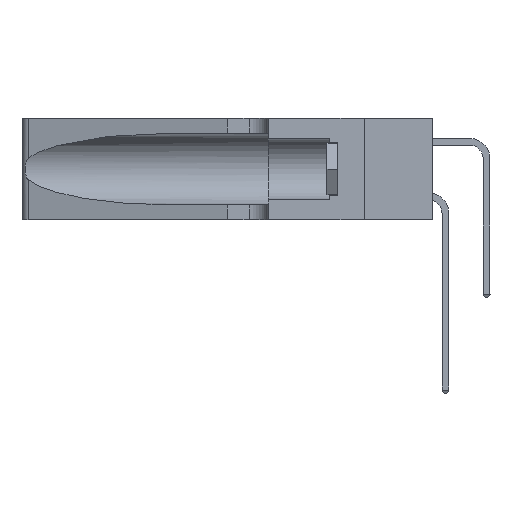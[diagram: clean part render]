
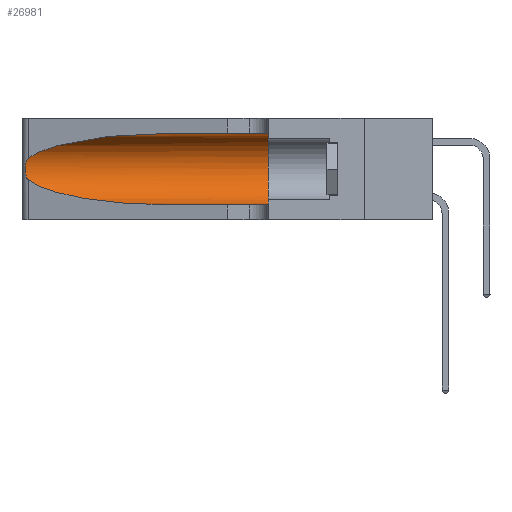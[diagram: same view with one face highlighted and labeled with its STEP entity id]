
A CAD part, left-side view. The second image highlights one B-rep face of the part: STEP entity #26981.
In plain terms, the highlighted cylindrical face has radius 3.308 mm (diameter 6.617 mm), a partial arc.
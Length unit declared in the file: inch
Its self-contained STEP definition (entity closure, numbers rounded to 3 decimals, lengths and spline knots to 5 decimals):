
#439 = CARTESIAN_POINT ( 'NONE',  ( 0.1305, 0.35, 0.185 ) ) ;
#847 = CARTESIAN_POINT ( 'NONE',  ( 0.25555, 1.22994, 0.2215 ) ) ;
#937 = CARTESIAN_POINT ( 'NONE',  ( 0.26017, 1.23833, 0.17102 ) ) ;
#1158 = CIRCLE ( 'NONE', #15803, 0.13025 ) ;
#1574 = CARTESIAN_POINT ( 'NONE',  ( 0.1305, 1.61858, 0.31525 ) ) ;
#1916 = CARTESIAN_POINT ( 'NONE',  ( 0.2373, 1.15595, 0.08982 ) ) ;
#1988 = ORIENTED_EDGE ( 'NONE', *, *, #2039, .T. ) ;
#2039 = EDGE_CURVE ( 'NONE', #26593, #8011, #4133, .T. ) ;
#2367 = ORIENTED_EDGE ( 'NONE', *, *, #3461, .T. ) ;
#2606 = EDGE_CURVE ( 'NONE', #6493, #22033, #1158, .T. ) ;
#2613 = DIRECTION ( 'NONE',  ( 0., 0., 1. ) ) ;
#2616 = CARTESIAN_POINT ( 'NONE',  ( 0.1305, 0.72297, 0.31525 ) ) ;
#3126 = CARTESIAN_POINT ( 'NONE',  ( 0.25789, 1.23486, 0.15765 ) ) ;
#3461 = EDGE_CURVE ( 'NONE', #25106, #22033, #8865, .T. ) ;
#4133 = B_SPLINE_CURVE_WITH_KNOTS ( 'NONE', 3,
 ( #22318, #847, #7370, #9510, #24423, #11702, #26543, #13853, #937, #15999, #3126, #18124, #5297, #20237 ),
 .UNSPECIFIED., .F., .F.,
 ( 4, 2, 2, 2, 2, 2, 4 ),
 ( 0., 0.00027, 0.00053, 0.00107, 0.0016, 0.00187, 0.00214 ),
 .UNSPECIFIED. ) ;
#4388 = ORIENTED_EDGE ( 'NONE', *, *, #7246, .T. ) ;
#4979 =( BOUNDED_CURVE ( )  B_SPLINE_CURVE ( 3, ( #8338, #1916, #19069, #6282 ),
 .UNSPECIFIED., .F., .F. ) 
 B_SPLINE_CURVE_WITH_KNOTS ( ( 4, 4 ),
 ( 3.44316, 4.71239 ),
 .UNSPECIFIED. ) 
 CURVE ( )  GEOMETRIC_REPRESENTATION_ITEM ( )  RATIONAL_B_SPLINE_CURVE ( ( 1., 0.87, 0.87, 1. ) ) 
 REPRESENTATION_ITEM ( '' )  );
#5297 = CARTESIAN_POINT ( 'NONE',  ( 0.25555, 1.22993, 0.14849 ) ) ;
#5604 = VECTOR ( 'NONE', #16625, 39.37008 ) ;
#5694 = CARTESIAN_POINT ( 'NONE',  ( 0.1305, 0.35, 0.05475 ) ) ;
#6282 = CARTESIAN_POINT ( 'NONE',  ( 0.1305, 0.72297, 0.05475 ) ) ;
#6493 = VERTEX_POINT ( 'NONE', #25666 ) ;
#6662 = AXIS2_PLACEMENT_3D ( 'NONE', #27594, #27686, #14990 ) ;
#7246 = EDGE_CURVE ( 'NONE', #23212, #26593, #12064, .T. ) ;
#7370 = CARTESIAN_POINT ( 'NONE',  ( 0.25639, 1.23184, 0.21858 ) ) ;
#8011 = VERTEX_POINT ( 'NONE', #9977 ) ;
#8197 = VECTOR ( 'NONE', #12387, 39.37008 ) ;
#8338 = CARTESIAN_POINT ( 'NONE',  ( 0.25487, 1.22718, 0.14631 ) ) ;
#8865 = LINE ( 'NONE', #10211, #8197 ) ;
#9374 = CARTESIAN_POINT ( 'NONE',  ( 0.25487, 1.22718, 0.22369 ) ) ;
#9510 = CARTESIAN_POINT ( 'NONE',  ( 0.25787, 1.23484, 0.2124 ) ) ;
#9977 = CARTESIAN_POINT ( 'NONE',  ( 0.25487, 1.22718, 0.14631 ) ) ;
#10211 = CARTESIAN_POINT ( 'NONE',  ( 0.1305, 1.61858, 0.05475 ) ) ;
#11135 = CARTESIAN_POINT ( 'NONE',  ( 0.2373, 1.15595, 0.28018 ) ) ;
#11506 = ORIENTED_EDGE ( 'NONE', *, *, #26190, .F. ) ;
#11702 = CARTESIAN_POINT ( 'NONE',  ( 0.26018, 1.23835, 0.19895 ) ) ;
#11724 = EDGE_CURVE ( 'NONE', #8011, #25106, #4979, .T. ) ;
#11952 = CYLINDRICAL_SURFACE ( 'NONE', #6662, 0.13025 ) ;
#12064 =( BOUNDED_CURVE ( )  B_SPLINE_CURVE ( 3, ( #21747, #23882, #11135, #25993 ),
 .UNSPECIFIED., .F., .F. ) 
 B_SPLINE_CURVE_WITH_KNOTS ( ( 4, 4 ),
 ( 1.5708, 2.84003 ),
 .UNSPECIFIED. ) 
 CURVE ( )  GEOMETRIC_REPRESENTATION_ITEM ( )  RATIONAL_B_SPLINE_CURVE ( ( 1., 0.87, 0.87, 1. ) ) 
 REPRESENTATION_ITEM ( '' )  );
#12387 = DIRECTION ( 'NONE',  ( 0., -1., 0. ) ) ;
#12666 = ORIENTED_EDGE ( 'NONE', *, *, #2606, .F. ) ;
#13853 = CARTESIAN_POINT ( 'NONE',  ( 0.26075, 1.23896, 0.178 ) ) ;
#14990 = DIRECTION ( 'NONE',  ( 0., 0., -1. ) ) ;
#15486 = DIRECTION ( 'NONE',  ( 0., 1., 0. ) ) ;
#15803 = AXIS2_PLACEMENT_3D ( 'NONE', #439, #15486, #2613 ) ;
#15999 = CARTESIAN_POINT ( 'NONE',  ( 0.25856, 1.23593, 0.16098 ) ) ;
#16625 = DIRECTION ( 'NONE',  ( 0., -1., 0. ) ) ;
#16942 = EDGE_LOOP ( 'NONE', ( #4388, #1988, #22375, #2367, #12666, #11506 ) ) ;
#17728 = CARTESIAN_POINT ( 'NONE',  ( 0.1305, 0.72297, 0.05475 ) ) ;
#18124 = CARTESIAN_POINT ( 'NONE',  ( 0.25639, 1.23186, 0.15144 ) ) ;
#19069 = CARTESIAN_POINT ( 'NONE',  ( 0.18966, 0.96281, 0.05475 ) ) ;
#20237 = CARTESIAN_POINT ( 'NONE',  ( 0.25487, 1.22718, 0.14631 ) ) ;
#20254 = FACE_OUTER_BOUND ( 'NONE', #16942, .T. ) ;
#21294 = LINE ( 'NONE', #1574, #5604 ) ;
#21747 = CARTESIAN_POINT ( 'NONE',  ( 0.1305, 0.72297, 0.31525 ) ) ;
#22033 = VERTEX_POINT ( 'NONE', #5694 ) ;
#22318 = CARTESIAN_POINT ( 'NONE',  ( 0.25487, 1.22718, 0.22369 ) ) ;
#22375 = ORIENTED_EDGE ( 'NONE', *, *, #11724, .T. ) ;
#23212 = VERTEX_POINT ( 'NONE', #2616 ) ;
#23882 = CARTESIAN_POINT ( 'NONE',  ( 0.18966, 0.96281, 0.31525 ) ) ;
#24423 = CARTESIAN_POINT ( 'NONE',  ( 0.25854, 1.2359, 0.20912 ) ) ;
#25106 = VERTEX_POINT ( 'NONE', #17728 ) ;
#25666 = CARTESIAN_POINT ( 'NONE',  ( 0.1305, 0.35, 0.31525 ) ) ;
#25993 = CARTESIAN_POINT ( 'NONE',  ( 0.25487, 1.22718, 0.22369 ) ) ;
#26190 = EDGE_CURVE ( 'NONE', #23212, #6493, #21294, .T. ) ;
#26543 = CARTESIAN_POINT ( 'NONE',  ( 0.26075, 1.23896, 0.19203 ) ) ;
#26593 = VERTEX_POINT ( 'NONE', #9374 ) ;
#26981 = ADVANCED_FACE ( 'NONE', ( #20254 ), #11952, .F. ) ;
#27594 = CARTESIAN_POINT ( 'NONE',  ( 0.1305, 1.61858, 0.185 ) ) ;
#27686 = DIRECTION ( 'NONE',  ( 0., -1., 0. ) ) ;
